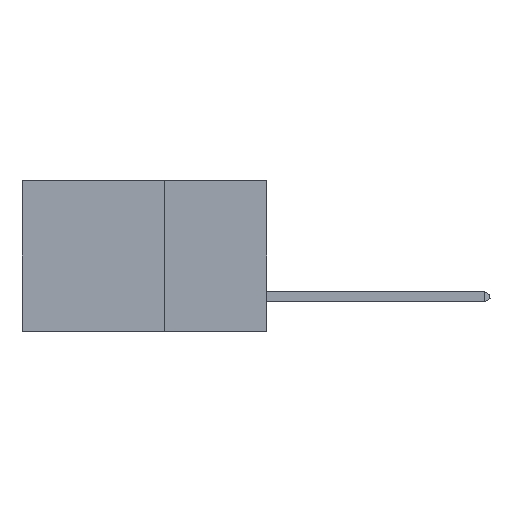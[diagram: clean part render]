
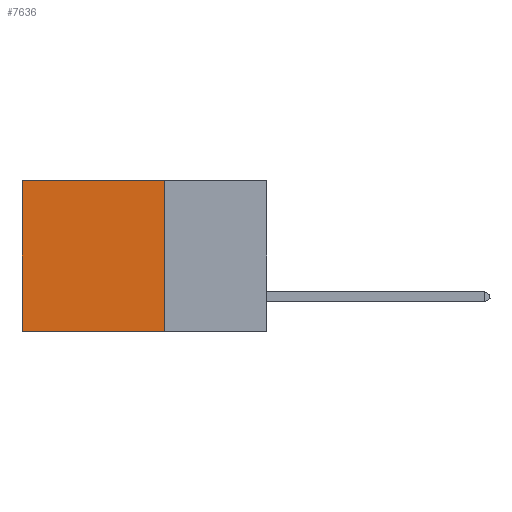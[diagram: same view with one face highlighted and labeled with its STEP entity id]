
A CAD part, left-side view. The second image highlights one B-rep face of the part: STEP entity #7636.
In plain terms, the highlighted planar face has unit normal (-1, 0, 0).
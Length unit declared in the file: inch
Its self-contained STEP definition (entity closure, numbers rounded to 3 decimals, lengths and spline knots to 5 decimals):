
#290 = EDGE_CURVE ( 'NONE', #12342, #4877, #6031, .T. ) ;
#502 = ORIENTED_EDGE ( 'NONE', *, *, #2480, .T. ) ;
#726 = LINE ( 'NONE', #16722, #2708 ) ;
#990 = CARTESIAN_POINT ( 'NONE',  ( 0.2875, 0.25, 0. ) ) ;
#1189 = EDGE_CURVE ( 'NONE', #15805, #4877, #12208, .T. ) ;
#1247 = ORIENTED_EDGE ( 'NONE', *, *, #290, .F. ) ;
#2014 = DIRECTION ( 'NONE',  ( 0., 0., -1. ) ) ;
#2205 = VECTOR ( 'NONE', #6310, 39.37008 ) ;
#2480 = EDGE_CURVE ( 'NONE', #14423, #15805, #726, .T. ) ;
#2571 = CARTESIAN_POINT ( 'NONE',  ( 0.2875, 0.6, 0. ) ) ;
#2702 = CARTESIAN_POINT ( 'NONE',  ( 0.2875, 0.25, -0.37 ) ) ;
#2708 = VECTOR ( 'NONE', #8101, 39.37008 ) ;
#3391 = PLANE ( 'NONE',  #4767 ) ;
#3441 = ORIENTED_EDGE ( 'NONE', *, *, #1189, .T. ) ;
#3616 = LINE ( 'NONE', #990, #16662 ) ;
#4107 = CARTESIAN_POINT ( 'NONE',  ( 0.2875, 0.6, 0. ) ) ;
#4689 = DIRECTION ( 'NONE',  ( 0., 0., -1. ) ) ;
#4767 = AXIS2_PLACEMENT_3D ( 'NONE', #6134, #14824, #4689 ) ;
#4815 = ORIENTED_EDGE ( 'NONE', *, *, #12684, .F. ) ;
#4877 = VERTEX_POINT ( 'NONE', #17266 ) ;
#6031 = LINE ( 'NONE', #12154, #2205 ) ;
#6134 = CARTESIAN_POINT ( 'NONE',  ( 0.2875, 0.25, 0. ) ) ;
#6310 = DIRECTION ( 'NONE',  ( 0., 1., 0. ) ) ;
#7498 = VECTOR ( 'NONE', #15364, 39.37008 ) ;
#7636 = ADVANCED_FACE ( 'NONE', ( #9847 ), #3391, .F. ) ;
#8101 = DIRECTION ( 'NONE',  ( 0., 1., 0. ) ) ;
#9847 = FACE_OUTER_BOUND ( 'NONE', #17594, .T. ) ;
#12154 = CARTESIAN_POINT ( 'NONE',  ( 0.2875, 0.25, -0.37 ) ) ;
#12208 = LINE ( 'NONE', #4107, #7498 ) ;
#12342 = VERTEX_POINT ( 'NONE', #2702 ) ;
#12684 = EDGE_CURVE ( 'NONE', #14423, #12342, #3616, .T. ) ;
#14423 = VERTEX_POINT ( 'NONE', #18073 ) ;
#14824 = DIRECTION ( 'NONE',  ( 1., 0., 0. ) ) ;
#15364 = DIRECTION ( 'NONE',  ( 0., 0., -1. ) ) ;
#15805 = VERTEX_POINT ( 'NONE', #2571 ) ;
#16662 = VECTOR ( 'NONE', #2014, 39.37008 ) ;
#16722 = CARTESIAN_POINT ( 'NONE',  ( 0.2875, 0.25, 0. ) ) ;
#17266 = CARTESIAN_POINT ( 'NONE',  ( 0.2875, 0.6, -0.37 ) ) ;
#17594 = EDGE_LOOP ( 'NONE', ( #3441, #1247, #4815, #502 ) ) ;
#18073 = CARTESIAN_POINT ( 'NONE',  ( 0.2875, 0.25, 0. ) ) ;
